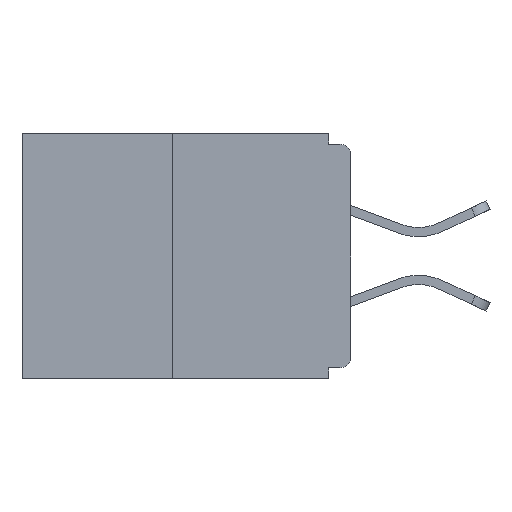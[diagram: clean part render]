
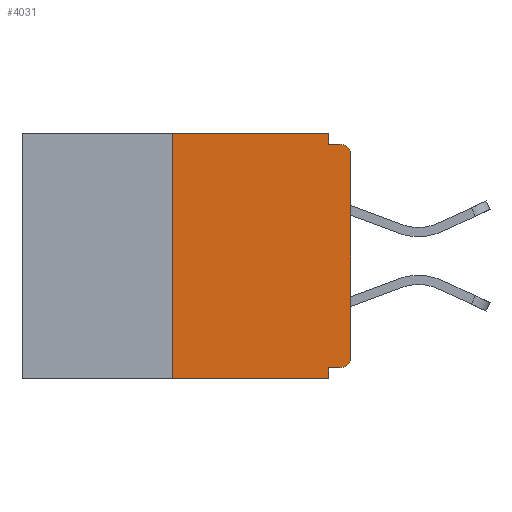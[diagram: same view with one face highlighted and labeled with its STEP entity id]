
A CAD part, left-side view. The second image highlights one B-rep face of the part: STEP entity #4031.
In plain terms, the highlighted planar face has unit normal (-1, 0, 0).
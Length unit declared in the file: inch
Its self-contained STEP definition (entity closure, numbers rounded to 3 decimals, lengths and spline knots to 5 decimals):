
#328 = VECTOR ( 'NONE', #8345, 39.37008 ) ;
#440 = ORIENTED_EDGE ( 'NONE', *, *, #8681, .T. ) ;
#455 = FACE_OUTER_BOUND ( 'NONE', #17843, .T. ) ;
#465 = VECTOR ( 'NONE', #16356, 39.37008 ) ;
#1058 = EDGE_CURVE ( 'NONE', #15530, #28920, #20062, .T. ) ;
#1251 = LINE ( 'NONE', #4106, #465 ) ;
#1387 = CARTESIAN_POINT ( 'NONE',  ( 0., 0.46, 0. ) ) ;
#1599 = PLANE ( 'NONE',  #14880 ) ;
#2647 = CARTESIAN_POINT ( 'NONE',  ( 0., 0., -0.313 ) ) ;
#3469 = CARTESIAN_POINT ( 'NONE',  ( 0., 0.25, -0.343 ) ) ;
#4031 = ADVANCED_FACE ( 'NONE', ( #455 ), #1599, .F. ) ;
#4106 = CARTESIAN_POINT ( 'NONE',  ( 0., 0., -0.328 ) ) ;
#4286 = CARTESIAN_POINT ( 'NONE',  ( 0., 0.031, -0.343 ) ) ;
#4288 = DIRECTION ( 'NONE',  ( 0., 0., -1. ) ) ;
#4291 = VERTEX_POINT ( 'NONE', #3469 ) ;
#4922 = DIRECTION ( 'NONE',  ( -1., 0., 0. ) ) ;
#5049 = LINE ( 'NONE', #23877, #30157 ) ;
#5402 = VERTEX_POINT ( 'NONE', #23103 ) ;
#5513 = LINE ( 'NONE', #7236, #31002 ) ;
#6031 = CARTESIAN_POINT ( 'NONE',  ( 0., 0.25, 0. ) ) ;
#6822 = VECTOR ( 'NONE', #9365, 39.37008 ) ;
#7122 = VECTOR ( 'NONE', #8892, 39.37008 ) ;
#7236 = CARTESIAN_POINT ( 'NONE',  ( 0., 0.25, 0. ) ) ;
#7658 = AXIS2_PLACEMENT_3D ( 'NONE', #19493, #4922, #10588 ) ;
#8077 = DIRECTION ( 'NONE',  ( 0., -1., 0. ) ) ;
#8222 = VERTEX_POINT ( 'NONE', #18127 ) ;
#8345 = DIRECTION ( 'NONE',  ( 0., -1., 0. ) ) ;
#8681 = EDGE_CURVE ( 'NONE', #12194, #14833, #23437, .T. ) ;
#8892 = DIRECTION ( 'NONE',  ( 0., 0., -1. ) ) ;
#9365 = DIRECTION ( 'NONE',  ( 0., 0., 1. ) ) ;
#9428 = ORIENTED_EDGE ( 'NONE', *, *, #28435, .T. ) ;
#9447 = EDGE_CURVE ( 'NONE', #4291, #29050, #5513, .T. ) ;
#9485 = VERTEX_POINT ( 'NONE', #19440 ) ;
#9779 = CARTESIAN_POINT ( 'NONE',  ( 0., 0.031, -0.015 ) ) ;
#9996 = VERTEX_POINT ( 'NONE', #21518 ) ;
#10049 = ORIENTED_EDGE ( 'NONE', *, *, #9447, .F. ) ;
#10082 = ORIENTED_EDGE ( 'NONE', *, *, #14314, .F. ) ;
#10588 = DIRECTION ( 'NONE',  ( 0., 0., -1. ) ) ;
#12194 = VERTEX_POINT ( 'NONE', #15742 ) ;
#12262 = EDGE_CURVE ( 'NONE', #14833, #9996, #31156, .T. ) ;
#13240 = LINE ( 'NONE', #4286, #7122 ) ;
#13566 = EDGE_CURVE ( 'NONE', #5402, #15530, #5049, .T. ) ;
#13616 = CARTESIAN_POINT ( 'NONE',  ( 0., 0.015, -0.015 ) ) ;
#13617 = CARTESIAN_POINT ( 'NONE',  ( 0., 0.015, -0.03 ) ) ;
#14221 = EDGE_CURVE ( 'NONE', #4291, #9485, #29734, .T. ) ;
#14314 = EDGE_CURVE ( 'NONE', #12194, #8222, #1251, .T. ) ;
#14387 = VECTOR ( 'NONE', #30612, 39.37008 ) ;
#14833 = VERTEX_POINT ( 'NONE', #2647 ) ;
#14880 = AXIS2_PLACEMENT_3D ( 'NONE', #1387, #30580, #21557 ) ;
#15530 = VERTEX_POINT ( 'NONE', #9779 ) ;
#15742 = CARTESIAN_POINT ( 'NONE',  ( 0., 0.015, -0.328 ) ) ;
#15883 = CARTESIAN_POINT ( 'NONE',  ( 0., 0., -0.015 ) ) ;
#16062 = DIRECTION ( 'NONE',  ( 0., 0., -1. ) ) ;
#16356 = DIRECTION ( 'NONE',  ( 0., 1., 0. ) ) ;
#17843 = EDGE_LOOP ( 'NONE', ( #23844, #10049, #22843, #27567, #10082, #440, #27616, #9428, #31153, #21757 ) ) ;
#18127 = CARTESIAN_POINT ( 'NONE',  ( 0., 0.031, -0.328 ) ) ;
#18277 = CIRCLE ( 'NONE', #26433, 0.015 ) ;
#19440 = CARTESIAN_POINT ( 'NONE',  ( 0., 0.031, -0.343 ) ) ;
#19493 = CARTESIAN_POINT ( 'NONE',  ( 0., 0.015, -0.313 ) ) ;
#20062 = LINE ( 'NONE', #15883, #14387 ) ;
#20085 = LINE ( 'NONE', #30423, #328 ) ;
#21518 = CARTESIAN_POINT ( 'NONE',  ( 0., 0., -0.03 ) ) ;
#21557 = DIRECTION ( 'NONE',  ( 0., 0., -1. ) ) ;
#21757 = ORIENTED_EDGE ( 'NONE', *, *, #13566, .F. ) ;
#22843 = ORIENTED_EDGE ( 'NONE', *, *, #14221, .T. ) ;
#23103 = CARTESIAN_POINT ( 'NONE',  ( 0., 0.031, 0. ) ) ;
#23307 = VECTOR ( 'NONE', #8077, 39.37008 ) ;
#23437 = CIRCLE ( 'NONE', #7658, 0.015 ) ;
#23443 = EDGE_CURVE ( 'NONE', #8222, #9485, #13240, .T. ) ;
#23844 = ORIENTED_EDGE ( 'NONE', *, *, #29506, .F. ) ;
#23877 = CARTESIAN_POINT ( 'NONE',  ( 0., 0.031, 0. ) ) ;
#25176 = CARTESIAN_POINT ( 'NONE',  ( 0., 0.46, -0.343 ) ) ;
#26433 = AXIS2_PLACEMENT_3D ( 'NONE', #13617, #30596, #16062 ) ;
#27567 = ORIENTED_EDGE ( 'NONE', *, *, #23443, .F. ) ;
#27616 = ORIENTED_EDGE ( 'NONE', *, *, #12262, .T. ) ;
#28435 = EDGE_CURVE ( 'NONE', #9996, #28920, #18277, .T. ) ;
#28467 = CARTESIAN_POINT ( 'NONE',  ( 0., 0., 0. ) ) ;
#28920 = VERTEX_POINT ( 'NONE', #13616 ) ;
#29050 = VERTEX_POINT ( 'NONE', #6031 ) ;
#29506 = EDGE_CURVE ( 'NONE', #29050, #5402, #20085, .T. ) ;
#29734 = LINE ( 'NONE', #25176, #23307 ) ;
#30157 = VECTOR ( 'NONE', #4288, 39.37008 ) ;
#30423 = CARTESIAN_POINT ( 'NONE',  ( 0., 0.46, 0. ) ) ;
#30580 = DIRECTION ( 'NONE',  ( 1., 0., 0. ) ) ;
#30596 = DIRECTION ( 'NONE',  ( -1., 0., 0. ) ) ;
#30612 = DIRECTION ( 'NONE',  ( 0., -1., 0. ) ) ;
#31002 = VECTOR ( 'NONE', #31361, 39.37008 ) ;
#31153 = ORIENTED_EDGE ( 'NONE', *, *, #1058, .F. ) ;
#31156 = LINE ( 'NONE', #28467, #6822 ) ;
#31361 = DIRECTION ( 'NONE',  ( 0., 0., 1. ) ) ;
